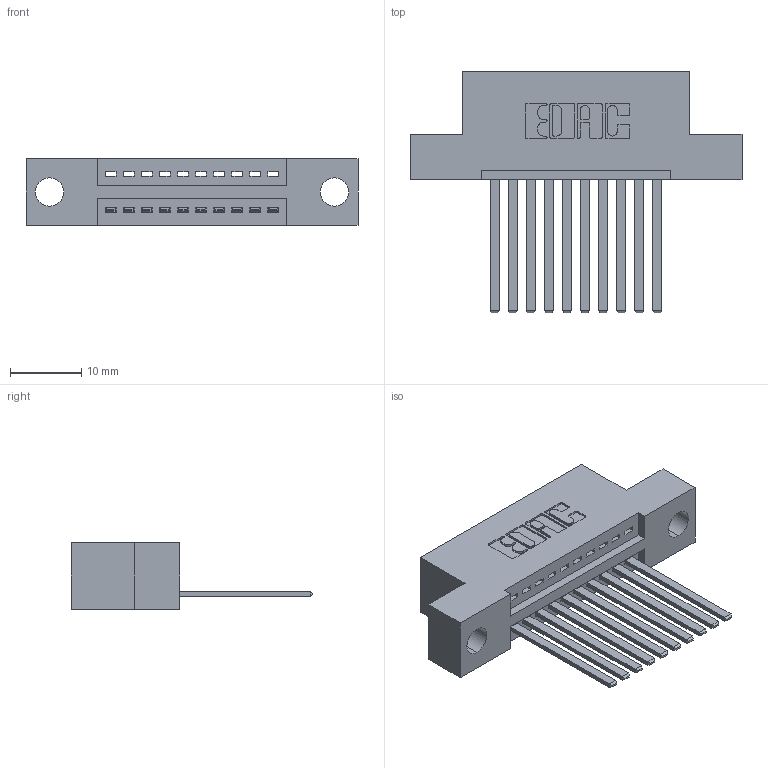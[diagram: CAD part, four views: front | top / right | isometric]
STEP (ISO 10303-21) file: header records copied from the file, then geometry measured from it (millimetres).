
FILE_DESCRIPTION (( 'STEP AP203' ), '1' );
FILE_NAME ('395-010-544-104.STEP', '2021-05-31T14:15:34', ( '' ), ( '' ), 'SwSTEP 2.0', 'SolidWorks 2020', '' );
FILE_SCHEMA (( 'CONFIG_CONTROL_DESIGN' ));
Length unit declared in the file: inch
Products named in the file (3): 395-010-544-104; 345-292-001_345-293-144; 345 Part_Flush Mounting Lugs - 0.156 Dia-TI
Assembly tree (11 placements, depth 2):
  395-010-544-104
    345 Part_Flush Mounting Lugs - 0.156 Dia-TI
    345-292-001_345-293-144  x10
Bounding box: 46.61 x 33.96 x 9.4 mm (x, y, z)
Volume: 4174.7 mm3; surface area: 5303 mm2
Topology: 11 solids, 11 shells, 660 faces, 1957 edges, 1290 vertices
Faces by surface type: plane 454, cylinder 206
Entity records: 12069 total; most frequent: CARTESIAN_POINT 2100, ORIENTED_EDGE 2042, DIRECTION 1877, EDGE_CURVE 1021, VECTOR 853, LINE 853, VERTEX_POINT 678, AXIS2_PLACEMENT_3D 512
